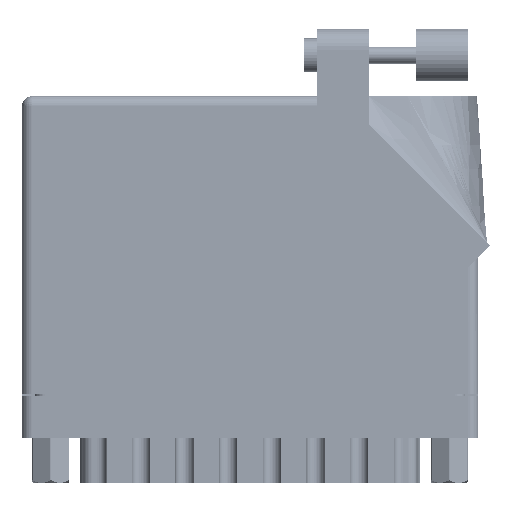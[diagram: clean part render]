
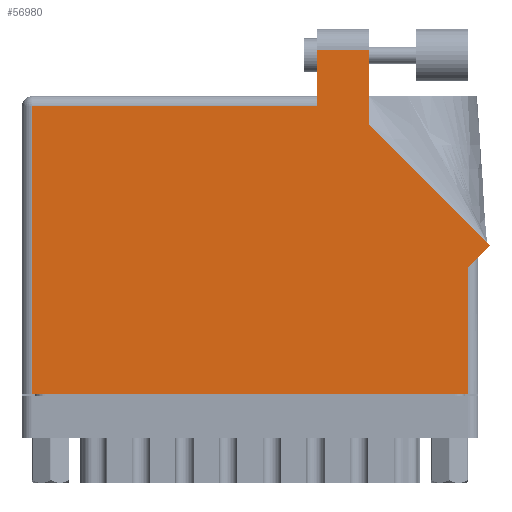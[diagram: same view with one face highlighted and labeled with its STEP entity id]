
A CAD part, front view. The second image highlights one B-rep face of the part: STEP entity #56980.
In plain terms, the highlighted face is planar.
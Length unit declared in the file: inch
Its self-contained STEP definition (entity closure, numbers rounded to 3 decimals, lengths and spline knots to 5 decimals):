
#1688 = DIRECTION ( 'NONE',  ( 0.707, 0.707, 0. ) ) ;
#3301 = VECTOR ( 'NONE', #72315, 39.37008 ) ;
#5020 = VECTOR ( 'NONE', #61133, 39.37008 ) ;
#6081 = CARTESIAN_POINT ( 'NONE',  ( 1.758, 1.713, 0. ) ) ;
#6145 = CARTESIAN_POINT ( 'NONE',  ( 2.065, 1.60942, 0. ) ) ;
#7150 = LINE ( 'NONE', #18396, #59231 ) ;
#13588 = EDGE_CURVE ( 'NONE', #34751, #27176, #40295, .T. ) ;
#16116 = ORIENTED_EDGE ( 'NONE', *, *, #69218, .T. ) ;
#18396 = CARTESIAN_POINT ( 'NONE',  ( 2.656, 0.815, 0. ) ) ;
#18840 = CARTESIAN_POINT ( 'NONE',  ( 1.758, 2.05, 0. ) ) ;
#21830 = CARTESIAN_POINT ( 'NONE',  ( 2.718, 0.815, 0. ) ) ;
#22319 = DIRECTION ( 'NONE',  ( 0., -1., 0. ) ) ;
#22702 = EDGE_CURVE ( 'NONE', #45438, #83898, #49665, .T. ) ;
#23347 = ORIENTED_EDGE ( 'NONE', *, *, #37244, .T. ) ;
#24239 = LINE ( 'NONE', #40010, #3301 ) ;
#24711 = VECTOR ( 'NONE', #72911, 39.37008 ) ;
#24858 = CARTESIAN_POINT ( 'NONE',  ( 0.062, 0., 0. ) ) ;
#25563 = LINE ( 'NONE', #29286, #73436 ) ;
#25986 = VERTEX_POINT ( 'NONE', #24858 ) ;
#27176 = VERTEX_POINT ( 'NONE', #67656 ) ;
#29286 = CARTESIAN_POINT ( 'NONE',  ( 0.062, 0., 0. ) ) ;
#29515 = ORIENTED_EDGE ( 'NONE', *, *, #56937, .T. ) ;
#29835 = FACE_OUTER_BOUND ( 'NONE', #61872, .T. ) ;
#29955 = LINE ( 'NONE', #76779, #61175 ) ;
#31950 = ORIENTED_EDGE ( 'NONE', *, *, #33316, .T. ) ;
#33316 = EDGE_CURVE ( 'NONE', #83898, #34751, #29955, .T. ) ;
#34167 = CARTESIAN_POINT ( 'NONE',  ( 2.78871, 0.88571, 0. ) ) ;
#34751 = VERTEX_POINT ( 'NONE', #61304 ) ;
#35180 = DIRECTION ( 'NONE',  ( 0., 0., -1. ) ) ;
#35749 = DIRECTION ( 'NONE',  ( -1., 0., 0. ) ) ;
#36544 = VERTEX_POINT ( 'NONE', #54363 ) ;
#37033 = ORIENTED_EDGE ( 'NONE', *, *, #41374, .T. ) ;
#37244 = EDGE_CURVE ( 'NONE', #25986, #36544, #57896, .T. ) ;
#37884 = VERTEX_POINT ( 'NONE', #6081 ) ;
#40010 = CARTESIAN_POINT ( 'NONE',  ( 0., 1.713, 0. ) ) ;
#40295 = LINE ( 'NONE', #18840, #51735 ) ;
#41374 = EDGE_CURVE ( 'NONE', #36544, #85763, #7150, .T. ) ;
#44000 = EDGE_CURVE ( 'NONE', #37884, #71873, #24239, .T. ) ;
#44603 = DIRECTION ( 'NONE',  ( 0., 1., 0. ) ) ;
#45438 = VERTEX_POINT ( 'NONE', #34167 ) ;
#47151 = ORIENTED_EDGE ( 'NONE', *, *, #13588, .T. ) ;
#47450 = VECTOR ( 'NONE', #59710, 39.37008 ) ;
#47778 = CARTESIAN_POINT ( 'NONE',  ( 1.758, 1.775, 0. ) ) ;
#48008 = CARTESIAN_POINT ( 'NONE',  ( 0., 1.775, 0. ) ) ;
#49266 = EDGE_CURVE ( 'NONE', #71873, #25986, #25563, .T. ) ;
#49665 = LINE ( 'NONE', #73189, #24711 ) ;
#51735 = VECTOR ( 'NONE', #78712, 39.37008 ) ;
#53565 = AXIS2_PLACEMENT_3D ( 'NONE', #48008, #35180, #35749 ) ;
#54363 = CARTESIAN_POINT ( 'NONE',  ( 2.656, 0., 0. ) ) ;
#56064 = LINE ( 'NONE', #47778, #5020 ) ;
#56937 = EDGE_CURVE ( 'NONE', #85763, #45438, #74061, .T. ) ;
#56980 = ADVANCED_FACE ( 'NONE', ( #29835 ), #68633, .F. ) ;
#57896 = LINE ( 'NONE', #73099, #47450 ) ;
#59231 = VECTOR ( 'NONE', #44603, 39.37008 ) ;
#59710 = DIRECTION ( 'NONE',  ( 1., 0., 0. ) ) ;
#61133 = DIRECTION ( 'NONE',  ( 0., -1., 0. ) ) ;
#61175 = VECTOR ( 'NONE', #83989, 39.37008 ) ;
#61304 = CARTESIAN_POINT ( 'NONE',  ( 2.065, 2.05, 0. ) ) ;
#61872 = EDGE_LOOP ( 'NONE', ( #31950, #47151, #16116, #81758, #64139, #23347, #37033, #29515, #83354 ) ) ;
#64139 = ORIENTED_EDGE ( 'NONE', *, *, #49266, .T. ) ;
#65705 = CARTESIAN_POINT ( 'NONE',  ( 2.656, 0.753, 0. ) ) ;
#67656 = CARTESIAN_POINT ( 'NONE',  ( 1.758, 2.05, 0. ) ) ;
#68633 = PLANE ( 'NONE',  #53565 ) ;
#69218 = EDGE_CURVE ( 'NONE', #27176, #37884, #56064, .T. ) ;
#71873 = VERTEX_POINT ( 'NONE', #85724 ) ;
#72315 = DIRECTION ( 'NONE',  ( -1., 0., 0. ) ) ;
#72911 = DIRECTION ( 'NONE',  ( -0.707, 0.707, 0. ) ) ;
#73099 = CARTESIAN_POINT ( 'NONE',  ( 0., 0., 0. ) ) ;
#73189 = CARTESIAN_POINT ( 'NONE',  ( 2.78871, 0.88571, 0. ) ) ;
#73436 = VECTOR ( 'NONE', #22319, 39.37008 ) ;
#74061 = LINE ( 'NONE', #21830, #79324 ) ;
#76779 = CARTESIAN_POINT ( 'NONE',  ( 2.065, 1.60942, 0. ) ) ;
#78712 = DIRECTION ( 'NONE',  ( -1., 0., 0. ) ) ;
#79324 = VECTOR ( 'NONE', #1688, 39.37008 ) ;
#81758 = ORIENTED_EDGE ( 'NONE', *, *, #44000, .T. ) ;
#83354 = ORIENTED_EDGE ( 'NONE', *, *, #22702, .T. ) ;
#83898 = VERTEX_POINT ( 'NONE', #6145 ) ;
#83989 = DIRECTION ( 'NONE',  ( 0., 1., 0. ) ) ;
#85724 = CARTESIAN_POINT ( 'NONE',  ( 0.062, 1.713, 0. ) ) ;
#85763 = VERTEX_POINT ( 'NONE', #65705 ) ;
